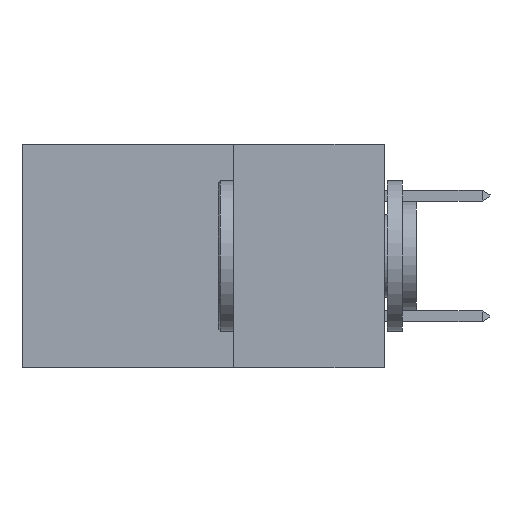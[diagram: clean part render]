
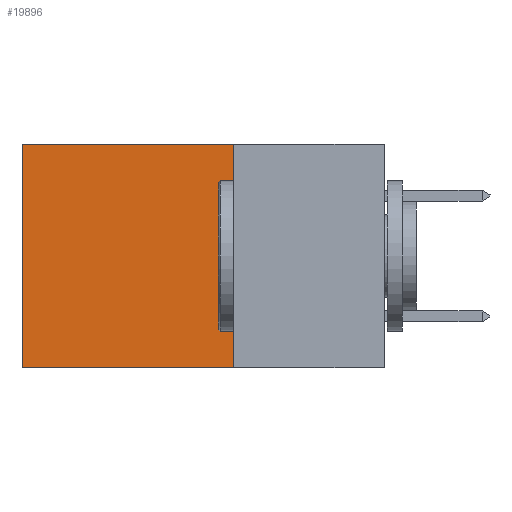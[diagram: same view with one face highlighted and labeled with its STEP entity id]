
A CAD part, left-side view. The second image highlights one B-rep face of the part: STEP entity #19896.
In plain terms, the highlighted planar face has unit normal (-1, 0, 0).
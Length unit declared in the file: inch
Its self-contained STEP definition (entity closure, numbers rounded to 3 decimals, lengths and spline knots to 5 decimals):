
#2088 = EDGE_CURVE ( 'NONE', #10787, #12902, #20313, .T. ) ;
#2207 = LINE ( 'NONE', #34647, #25868 ) ;
#3617 = CARTESIAN_POINT ( 'NONE',  ( 0.2875, 0.25, 0. ) ) ;
#5273 = CARTESIAN_POINT ( 'NONE',  ( 0.2875, 0.25, 0. ) ) ;
#7251 = EDGE_CURVE ( 'NONE', #12796, #33574, #2207, .T. ) ;
#7446 = AXIS2_PLACEMENT_3D ( 'NONE', #7634, #32060, #34742 ) ;
#7586 = ORIENTED_EDGE ( 'NONE', *, *, #7251, .T. ) ;
#7634 = CARTESIAN_POINT ( 'NONE',  ( 0.2875, 0.25, 0. ) ) ;
#8700 = DIRECTION ( 'NONE',  ( 0., 0., -1. ) ) ;
#8836 = DIRECTION ( 'NONE',  ( 0., 0., -1. ) ) ;
#9414 = DIRECTION ( 'NONE',  ( 0., 1., 0. ) ) ;
#10787 = VERTEX_POINT ( 'NONE', #3617 ) ;
#10889 = LINE ( 'NONE', #5273, #32528 ) ;
#10938 = DIRECTION ( 'NONE',  ( 0., 1., 0. ) ) ;
#12796 = VERTEX_POINT ( 'NONE', #30516 ) ;
#12902 = VERTEX_POINT ( 'NONE', #33532 ) ;
#15467 = EDGE_LOOP ( 'NONE', ( #7586, #23195, #29855, #19685 ) ) ;
#17600 = CARTESIAN_POINT ( 'NONE',  ( 0.2875, 0.6, -0.37 ) ) ;
#19685 = ORIENTED_EDGE ( 'NONE', *, *, #29316, .T. ) ;
#19896 = ADVANCED_FACE ( 'NONE', ( #23207 ), #23834, .F. ) ;
#20313 = LINE ( 'NONE', #32783, #22403 ) ;
#21262 = CARTESIAN_POINT ( 'NONE',  ( 0.2875, 0.25, -0.37 ) ) ;
#22328 = LINE ( 'NONE', #21262, #25313 ) ;
#22403 = VECTOR ( 'NONE', #8836, 39.37008 ) ;
#23195 = ORIENTED_EDGE ( 'NONE', *, *, #33572, .F. ) ;
#23207 = FACE_OUTER_BOUND ( 'NONE', #15467, .T. ) ;
#23834 = PLANE ( 'NONE',  #7446 ) ;
#25313 = VECTOR ( 'NONE', #9414, 39.37008 ) ;
#25868 = VECTOR ( 'NONE', #8700, 39.37008 ) ;
#29316 = EDGE_CURVE ( 'NONE', #10787, #12796, #10889, .T. ) ;
#29855 = ORIENTED_EDGE ( 'NONE', *, *, #2088, .F. ) ;
#30516 = CARTESIAN_POINT ( 'NONE',  ( 0.2875, 0.6, 0. ) ) ;
#32060 = DIRECTION ( 'NONE',  ( 1., 0., 0. ) ) ;
#32528 = VECTOR ( 'NONE', #10938, 39.37008 ) ;
#32783 = CARTESIAN_POINT ( 'NONE',  ( 0.2875, 0.25, 0. ) ) ;
#33532 = CARTESIAN_POINT ( 'NONE',  ( 0.2875, 0.25, -0.37 ) ) ;
#33572 = EDGE_CURVE ( 'NONE', #12902, #33574, #22328, .T. ) ;
#33574 = VERTEX_POINT ( 'NONE', #17600 ) ;
#34647 = CARTESIAN_POINT ( 'NONE',  ( 0.2875, 0.6, 0. ) ) ;
#34742 = DIRECTION ( 'NONE',  ( 0., 0., -1. ) ) ;
